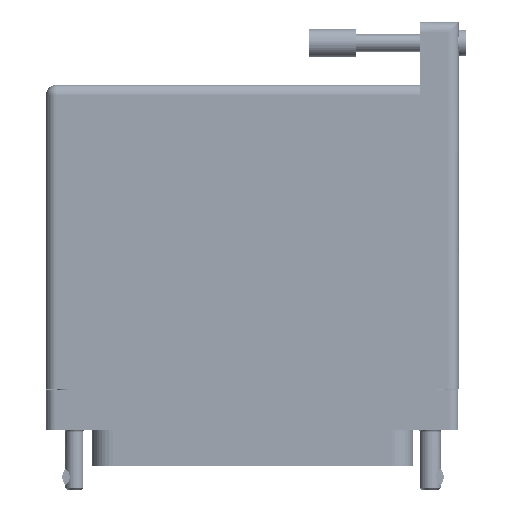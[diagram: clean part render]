
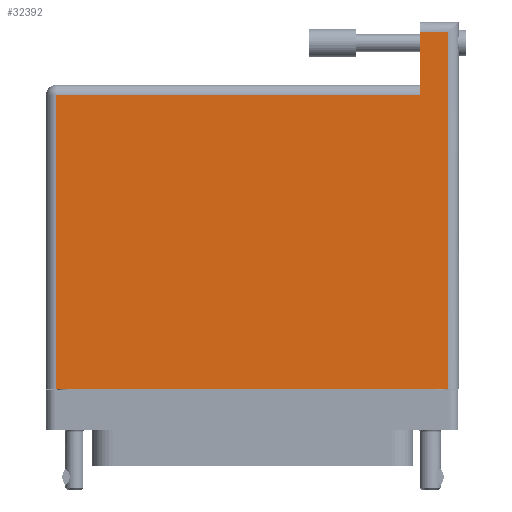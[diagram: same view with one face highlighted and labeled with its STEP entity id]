
A CAD part, front view. The second image highlights one B-rep face of the part: STEP entity #32392.
In plain terms, the highlighted face is planar.
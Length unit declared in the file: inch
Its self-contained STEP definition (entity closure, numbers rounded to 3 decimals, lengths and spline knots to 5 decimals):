
#2364 = VERTEX_POINT ( 'NONE', #95218 ) ;
#2457 = CARTESIAN_POINT ( 'NONE',  ( 1.1215, 2.35, 0.765 ) ) ;
#5626 = EDGE_CURVE ( 'NONE', #2364, #27322, #46748, .T. ) ;
#7900 = DIRECTION ( 'NONE',  ( -1., 0., 0. ) ) ;
#10165 = DIRECTION ( 'NONE',  ( -1., 0., 0. ) ) ;
#11688 = LINE ( 'NONE', #41665, #101230 ) ;
#15288 = ORIENTED_EDGE ( 'NONE', *, *, #17358, .T. ) ;
#17358 = EDGE_CURVE ( 'NONE', #71569, #51051, #73642, .T. ) ;
#17850 = DIRECTION ( 'NONE',  ( 0., 0., -1. ) ) ;
#17865 = ORIENTED_EDGE ( 'NONE', *, *, #80510, .T. ) ;
#25003 = CARTESIAN_POINT ( 'NONE',  ( -1.3775, -0.1, 0.765 ) ) ;
#25626 = CARTESIAN_POINT ( 'NONE',  ( 1.1215, 2.28, 0.765 ) ) ;
#26717 = VERTEX_POINT ( 'NONE', #50361 ) ;
#27322 = VERTEX_POINT ( 'NONE', #51960 ) ;
#27727 = DIRECTION ( 'NONE',  ( -1., 0., 0. ) ) ;
#32392 = ADVANCED_FACE ( 'NONE', ( #55440 ), #89401, .F. ) ;
#32639 = DIRECTION ( 'NONE',  ( 1., 0., 0. ) ) ;
#36741 = VECTOR ( 'NONE', #32639, 39.37008 ) ;
#41665 = CARTESIAN_POINT ( 'NONE',  ( -1.3775, 2.28, 0.765 ) ) ;
#42594 = VECTOR ( 'NONE', #99673, 39.37008 ) ;
#43739 = CARTESIAN_POINT ( 'NONE',  ( 1.3075, 2.35, 0.765 ) ) ;
#43807 = ORIENTED_EDGE ( 'NONE', *, *, #66517, .T. ) ;
#44502 = VECTOR ( 'NONE', #7900, 39.37008 ) ;
#46748 = LINE ( 'NONE', #25003, #36741 ) ;
#47928 = VECTOR ( 'NONE', #70813, 39.37008 ) ;
#49394 = CARTESIAN_POINT ( 'NONE',  ( -1.3775, 1.93, 0.765 ) ) ;
#50361 = CARTESIAN_POINT ( 'NONE',  ( 1.3075, 2.28, 0.765 ) ) ;
#51051 = VERTEX_POINT ( 'NONE', #90721 ) ;
#51610 = LINE ( 'NONE', #55195, #47928 ) ;
#51960 = CARTESIAN_POINT ( 'NONE',  ( 1.3075, -0.1, 0.765 ) ) ;
#55195 = CARTESIAN_POINT ( 'NONE',  ( -1.3075, -0.1, 0.765 ) ) ;
#55440 = FACE_OUTER_BOUND ( 'NONE', #89645, .T. ) ;
#59258 = VERTEX_POINT ( 'NONE', #101990 ) ;
#59309 = ORIENTED_EDGE ( 'NONE', *, *, #88320, .T. ) ;
#60576 = ORIENTED_EDGE ( 'NONE', *, *, #85568, .T. ) ;
#65071 = VECTOR ( 'NONE', #73986, 39.37008 ) ;
#66517 = EDGE_CURVE ( 'NONE', #26717, #71569, #11688, .T. ) ;
#70813 = DIRECTION ( 'NONE',  ( 0., -1., 0. ) ) ;
#71540 = AXIS2_PLACEMENT_3D ( 'NONE', #49394, #17850, #10165 ) ;
#71569 = VERTEX_POINT ( 'NONE', #25626 ) ;
#73642 = LINE ( 'NONE', #2457, #65071 ) ;
#73986 = DIRECTION ( 'NONE',  ( 0., -1., 0. ) ) ;
#80510 = EDGE_CURVE ( 'NONE', #51051, #59258, #99116, .T. ) ;
#85568 = EDGE_CURVE ( 'NONE', #59258, #2364, #51610, .T. ) ;
#87438 = CARTESIAN_POINT ( 'NONE',  ( -1.3775, 1.86, 0.765 ) ) ;
#88320 = EDGE_CURVE ( 'NONE', #27322, #26717, #92376, .T. ) ;
#89401 = PLANE ( 'NONE',  #71540 ) ;
#89645 = EDGE_LOOP ( 'NONE', ( #15288, #17865, #60576, #97336, #59309, #43807 ) ) ;
#90721 = CARTESIAN_POINT ( 'NONE',  ( 1.1215, 1.86, 0.765 ) ) ;
#92376 = LINE ( 'NONE', #43739, #42594 ) ;
#95218 = CARTESIAN_POINT ( 'NONE',  ( -1.3075, -0.1, 0.765 ) ) ;
#97336 = ORIENTED_EDGE ( 'NONE', *, *, #5626, .T. ) ;
#99116 = LINE ( 'NONE', #87438, #44502 ) ;
#99673 = DIRECTION ( 'NONE',  ( 0., 1., 0. ) ) ;
#101230 = VECTOR ( 'NONE', #27727, 39.37008 ) ;
#101990 = CARTESIAN_POINT ( 'NONE',  ( -1.3075, 1.86, 0.765 ) ) ;
